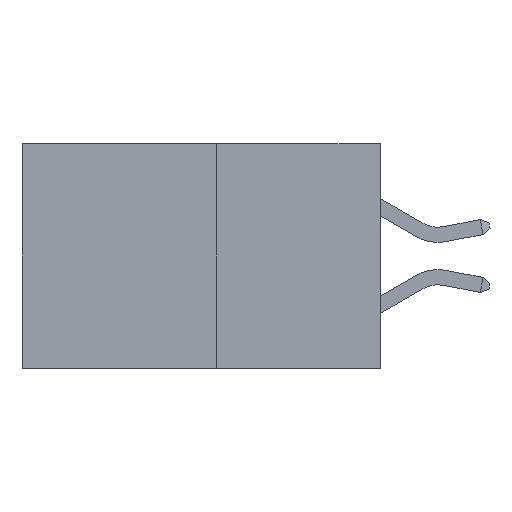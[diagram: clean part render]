
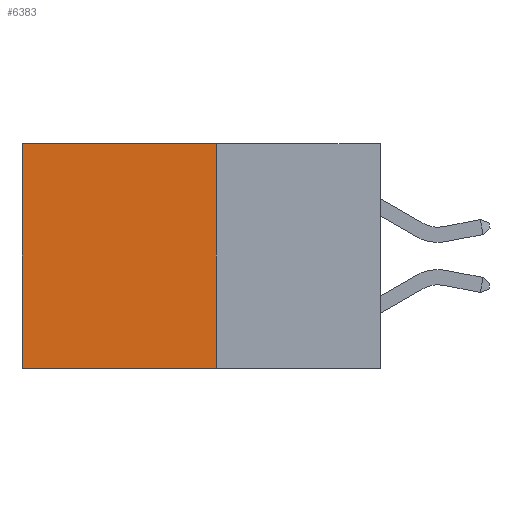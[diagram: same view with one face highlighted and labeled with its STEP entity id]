
A CAD part, left-side view. The second image highlights one B-rep face of the part: STEP entity #6383.
In plain terms, the highlighted planar face has unit normal (-1, 0, 0).
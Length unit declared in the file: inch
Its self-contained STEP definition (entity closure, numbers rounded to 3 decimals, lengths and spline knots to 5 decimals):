
#173 = ORIENTED_EDGE ( 'NONE', *, *, #8087, .F. ) ;
#178 = DIRECTION ( 'NONE',  ( 0., 0., -1. ) ) ;
#207 = ORIENTED_EDGE ( 'NONE', *, *, #7758, .T. ) ;
#352 = EDGE_CURVE ( 'NONE', #4136, #4840, #465, .T. ) ;
#430 = FACE_OUTER_BOUND ( 'NONE', #3329, .T. ) ;
#439 = ORIENTED_EDGE ( 'NONE', *, *, #352, .T. ) ;
#465 = LINE ( 'NONE', #2832, #2582 ) ;
#959 = VECTOR ( 'NONE', #3822, 39.37008 ) ;
#2153 = CARTESIAN_POINT ( 'NONE',  ( 0.277, 0.59, 0. ) ) ;
#2249 = DIRECTION ( 'NONE',  ( 0., 0., -1. ) ) ;
#2438 = ORIENTED_EDGE ( 'NONE', *, *, #5551, .F. ) ;
#2582 = VECTOR ( 'NONE', #2881, 39.37008 ) ;
#2832 = CARTESIAN_POINT ( 'NONE',  ( 0.277, 0.59, -0.37 ) ) ;
#2881 = DIRECTION ( 'NONE',  ( 0., 0., -1. ) ) ;
#3329 = EDGE_LOOP ( 'NONE', ( #439, #2438, #173, #207 ) ) ;
#3459 = CARTESIAN_POINT ( 'NONE',  ( 0.277, 0.59, -0.37 ) ) ;
#3706 = CARTESIAN_POINT ( 'NONE',  ( 0.277, 0.27, -0.37 ) ) ;
#3822 = DIRECTION ( 'NONE',  ( 0., 1., 0. ) ) ;
#3956 = VECTOR ( 'NONE', #6536, 39.37008 ) ;
#4125 = LINE ( 'NONE', #6939, #7601 ) ;
#4136 = VERTEX_POINT ( 'NONE', #2153 ) ;
#4455 = VERTEX_POINT ( 'NONE', #3706 ) ;
#4540 = CARTESIAN_POINT ( 'NONE',  ( 0.277, 0.27, 0. ) ) ;
#4840 = VERTEX_POINT ( 'NONE', #3459 ) ;
#5551 = EDGE_CURVE ( 'NONE', #4455, #4840, #5775, .T. ) ;
#5775 = LINE ( 'NONE', #6246, #3956 ) ;
#6246 = CARTESIAN_POINT ( 'NONE',  ( 0.277, 0.27, -0.37 ) ) ;
#6383 = ADVANCED_FACE ( 'NONE', ( #430 ), #6662, .F. ) ;
#6536 = DIRECTION ( 'NONE',  ( 0., 1., 0. ) ) ;
#6606 = DIRECTION ( 'NONE',  ( 1., 0., 0. ) ) ;
#6619 = AXIS2_PLACEMENT_3D ( 'NONE', #6655, #6606, #178 ) ;
#6655 = CARTESIAN_POINT ( 'NONE',  ( 0.277, 0.27, -0.37 ) ) ;
#6662 = PLANE ( 'NONE',  #6619 ) ;
#6939 = CARTESIAN_POINT ( 'NONE',  ( 0.277, 0.27, -0.37 ) ) ;
#7139 = CARTESIAN_POINT ( 'NONE',  ( 0.277, 0.27, 0. ) ) ;
#7601 = VECTOR ( 'NONE', #2249, 39.37008 ) ;
#7758 = EDGE_CURVE ( 'NONE', #8377, #4136, #8062, .T. ) ;
#8062 = LINE ( 'NONE', #7139, #959 ) ;
#8087 = EDGE_CURVE ( 'NONE', #8377, #4455, #4125, .T. ) ;
#8377 = VERTEX_POINT ( 'NONE', #4540 ) ;
